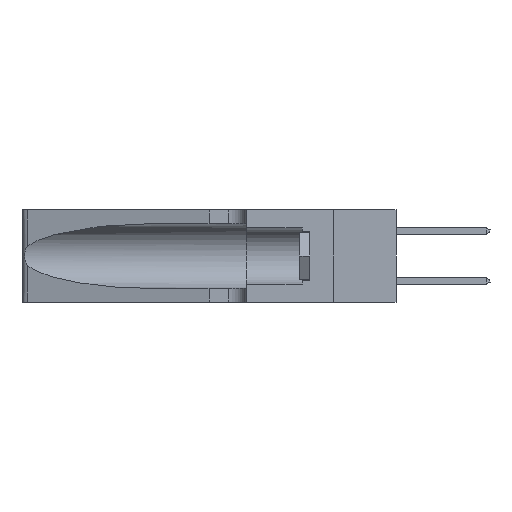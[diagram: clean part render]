
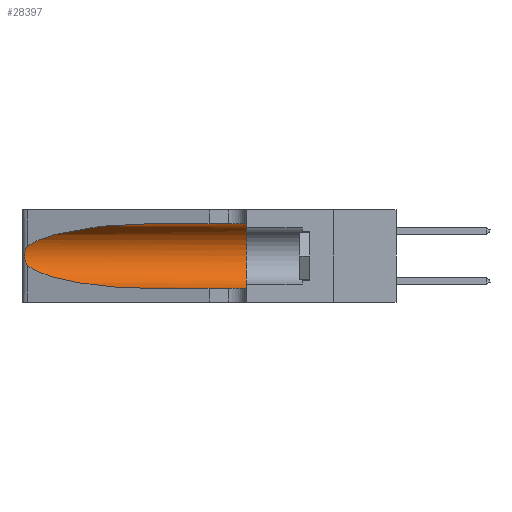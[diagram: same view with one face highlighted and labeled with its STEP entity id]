
A CAD part, left-side view. The second image highlights one B-rep face of the part: STEP entity #28397.
In plain terms, the highlighted cylindrical face has radius 3.308 mm (diameter 6.617 mm), a partial arc.
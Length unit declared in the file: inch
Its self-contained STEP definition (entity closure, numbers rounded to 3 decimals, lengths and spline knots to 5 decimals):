
#270 = ORIENTED_EDGE ( 'NONE', *, *, #15126, .F. ) ;
#445 = CARTESIAN_POINT ( 'NONE',  ( 0.25639, 1.23184, 0.21858 ) ) ;
#552 = CARTESIAN_POINT ( 'NONE',  ( 0.25789, 1.23486, 0.15765 ) ) ;
#1124 = LINE ( 'NONE', #3466, #12699 ) ;
#1318 = CARTESIAN_POINT ( 'NONE',  ( 0.18966, 0.96281, 0.05475 ) ) ;
#1464 = CARTESIAN_POINT ( 'NONE',  ( 0.1305, 0.35, 0.31525 ) ) ;
#2658 = CARTESIAN_POINT ( 'NONE',  ( 0.25487, 1.22718, 0.22369 ) ) ;
#2882 = CARTESIAN_POINT ( 'NONE',  ( 0.25555, 1.22993, 0.14849 ) ) ;
#3466 = CARTESIAN_POINT ( 'NONE',  ( 0.1305, 1.61858, 0.31525 ) ) ;
#3953 = VERTEX_POINT ( 'NONE', #24862 ) ;
#4728 = FACE_OUTER_BOUND ( 'NONE', #28369, .T. ) ;
#5681 = ORIENTED_EDGE ( 'NONE', *, *, #23681, .T. ) ;
#5832 = DIRECTION ( 'NONE',  ( 0., -1., 0. ) ) ;
#5888 = ORIENTED_EDGE ( 'NONE', *, *, #6371, .T. ) ;
#6371 = EDGE_CURVE ( 'NONE', #3953, #18763, #17644, .T. ) ;
#7480 = CARTESIAN_POINT ( 'NONE',  ( 0.25787, 1.23484, 0.2124 ) ) ;
#8493 = CARTESIAN_POINT ( 'NONE',  ( 0.1305, 0.35, 0.185 ) ) ;
#9842 = CARTESIAN_POINT ( 'NONE',  ( 0.26018, 1.23835, 0.19895 ) ) ;
#10238 = DIRECTION ( 'NONE',  ( 0., -1., 0. ) ) ;
#10512 = CARTESIAN_POINT ( 'NONE',  ( 0.1305, 1.61858, 0.185 ) ) ;
#10809 = DIRECTION ( 'NONE',  ( 0., 0., 1. ) ) ;
#11687 = VECTOR ( 'NONE', #10238, 39.37008 ) ;
#11909 = ORIENTED_EDGE ( 'NONE', *, *, #18188, .F. ) ;
#12106 = CARTESIAN_POINT ( 'NONE',  ( 0.26075, 1.23896, 0.178 ) ) ;
#12699 = VECTOR ( 'NONE', #12755, 39.37008 ) ;
#12755 = DIRECTION ( 'NONE',  ( 0., -1., 0. ) ) ;
#12849 = CARTESIAN_POINT ( 'NONE',  ( 0.25487, 1.22718, 0.14631 ) ) ;
#13030 = CARTESIAN_POINT ( 'NONE',  ( 0.25487, 1.22718, 0.14631 ) ) ;
#13877 = CARTESIAN_POINT ( 'NONE',  ( 0.25487, 1.22718, 0.22369 ) ) ;
#14372 = CARTESIAN_POINT ( 'NONE',  ( 0.25856, 1.23593, 0.16098 ) ) ;
#14451 = VERTEX_POINT ( 'NONE', #1464 ) ;
#14457 = AXIS2_PLACEMENT_3D ( 'NONE', #10512, #5832, #26109 ) ;
#15124 = CARTESIAN_POINT ( 'NONE',  ( 0.2373, 1.15595, 0.08982 ) ) ;
#15126 = EDGE_CURVE ( 'NONE', #14451, #18763, #19438, .T. ) ;
#15792 = VERTEX_POINT ( 'NONE', #17430 ) ;
#16391 = CARTESIAN_POINT ( 'NONE',  ( 0.2373, 1.15595, 0.28018 ) ) ;
#16614 = CARTESIAN_POINT ( 'NONE',  ( 0.25639, 1.23186, 0.15144 ) ) ;
#17039 = CARTESIAN_POINT ( 'NONE',  ( 0.1305, 0.35, 0.05475 ) ) ;
#17360 = CARTESIAN_POINT ( 'NONE',  ( 0.1305, 0.72297, 0.05475 ) ) ;
#17430 = CARTESIAN_POINT ( 'NONE',  ( 0.1305, 0.72297, 0.31525 ) ) ;
#17644 = LINE ( 'NONE', #21393, #11687 ) ;
#18188 = EDGE_CURVE ( 'NONE', #15792, #14451, #1124, .T. ) ;
#18763 = VERTEX_POINT ( 'NONE', #17039 ) ;
#18851 = CARTESIAN_POINT ( 'NONE',  ( 0.25487, 1.22718, 0.14631 ) ) ;
#19290 = EDGE_CURVE ( 'NONE', #28042, #27172, #26083, .T. ) ;
#19438 = CIRCLE ( 'NONE', #24414, 0.13025 ) ;
#20134 = ORIENTED_EDGE ( 'NONE', *, *, #19290, .T. ) ;
#20998 = CARTESIAN_POINT ( 'NONE',  ( 0.25487, 1.22718, 0.22369 ) ) ;
#21393 = CARTESIAN_POINT ( 'NONE',  ( 0.1305, 1.61858, 0.05475 ) ) ;
#22112 = CYLINDRICAL_SURFACE ( 'NONE', #14457, 0.13025 ) ;
#23124 = CARTESIAN_POINT ( 'NONE',  ( 0.25555, 1.22994, 0.2215 ) ) ;
#23221 = CARTESIAN_POINT ( 'NONE',  ( 0.25854, 1.2359, 0.20912 ) ) ;
#23681 = EDGE_CURVE ( 'NONE', #15792, #28042, #25352, .T. ) ;
#23937 = EDGE_CURVE ( 'NONE', #27172, #3953, #24820, .T. ) ;
#24167 = DIRECTION ( 'NONE',  ( 0., 1., 0. ) ) ;
#24414 = AXIS2_PLACEMENT_3D ( 'NONE', #8493, #24167, #10809 ) ;
#24820 =( BOUNDED_CURVE ( )  B_SPLINE_CURVE ( 3, ( #12849, #15124, #1318, #17360 ),
 .UNSPECIFIED., .F., .F. ) 
 B_SPLINE_CURVE_WITH_KNOTS ( ( 4, 4 ),
 ( 3.44316, 4.71239 ),
 .UNSPECIFIED. ) 
 CURVE ( )  GEOMETRIC_REPRESENTATION_ITEM ( )  RATIONAL_B_SPLINE_CURVE ( ( 1., 0.87, 0.87, 1. ) ) 
 REPRESENTATION_ITEM ( '' )  );
#24862 = CARTESIAN_POINT ( 'NONE',  ( 0.1305, 0.72297, 0.05475 ) ) ;
#25216 = CARTESIAN_POINT ( 'NONE',  ( 0.1305, 0.72297, 0.31525 ) ) ;
#25352 =( BOUNDED_CURVE ( )  B_SPLINE_CURVE ( 3, ( #25216, #27448, #16391, #2658 ),
 .UNSPECIFIED., .F., .F. ) 
 B_SPLINE_CURVE_WITH_KNOTS ( ( 4, 4 ),
 ( 1.5708, 2.84003 ),
 .UNSPECIFIED. ) 
 CURVE ( )  GEOMETRIC_REPRESENTATION_ITEM ( )  RATIONAL_B_SPLINE_CURVE ( ( 1., 0.87, 0.87, 1. ) ) 
 REPRESENTATION_ITEM ( '' )  );
#25446 = CARTESIAN_POINT ( 'NONE',  ( 0.26075, 1.23896, 0.19203 ) ) ;
#26083 = B_SPLINE_CURVE_WITH_KNOTS ( 'NONE', 3,
 ( #20998, #23124, #445, #7480, #23221, #9842, #25446, #12106, #27663, #14372, #552, #16614, #2882, #18851 ),
 .UNSPECIFIED., .F., .F.,
 ( 4, 2, 2, 2, 2, 2, 4 ),
 ( 0., 0.00027, 0.00053, 0.00107, 0.0016, 0.00187, 0.00214 ),
 .UNSPECIFIED. ) ;
#26109 = DIRECTION ( 'NONE',  ( 0., 0., -1. ) ) ;
#27172 = VERTEX_POINT ( 'NONE', #13030 ) ;
#27448 = CARTESIAN_POINT ( 'NONE',  ( 0.18966, 0.96281, 0.31525 ) ) ;
#27663 = CARTESIAN_POINT ( 'NONE',  ( 0.26017, 1.23833, 0.17102 ) ) ;
#28042 = VERTEX_POINT ( 'NONE', #13877 ) ;
#28143 = ORIENTED_EDGE ( 'NONE', *, *, #23937, .T. ) ;
#28369 = EDGE_LOOP ( 'NONE', ( #5681, #20134, #28143, #5888, #270, #11909 ) ) ;
#28397 = ADVANCED_FACE ( 'NONE', ( #4728 ), #22112, .F. ) ;
